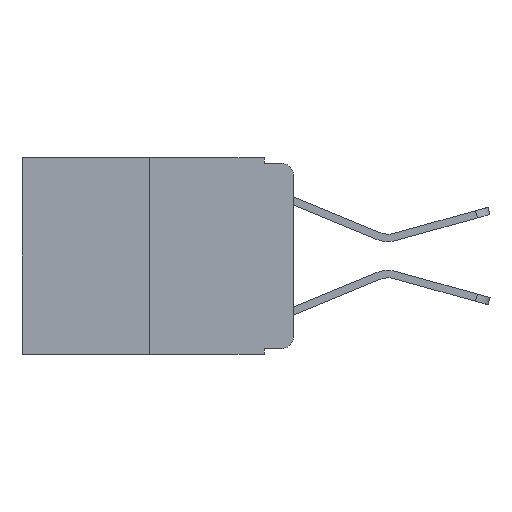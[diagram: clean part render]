
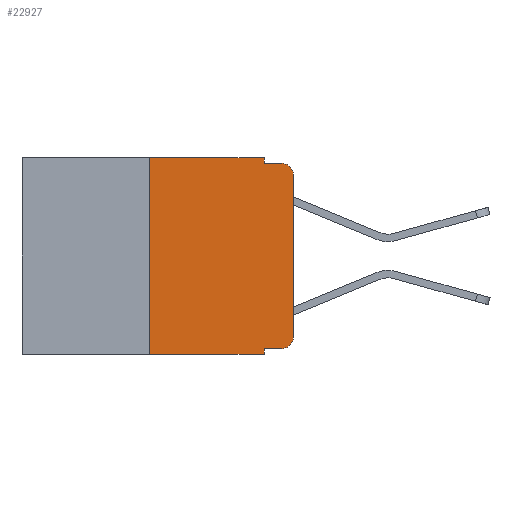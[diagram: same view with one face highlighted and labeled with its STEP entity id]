
A CAD part, left-side view. The second image highlights one B-rep face of the part: STEP entity #22927.
In plain terms, the highlighted planar face has unit normal (-1, 0, 0).
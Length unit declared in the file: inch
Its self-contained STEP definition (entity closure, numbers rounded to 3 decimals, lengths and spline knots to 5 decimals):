
#206 = EDGE_CURVE ( 'NONE', #16278, #2277, #17409, .T. ) ;
#449 = AXIS2_PLACEMENT_3D ( 'NONE', #2134, #2298, #22669 ) ;
#471 = ORIENTED_EDGE ( 'NONE', *, *, #9997, .T. ) ;
#782 = DIRECTION ( 'NONE',  ( 0., -1., 0. ) ) ;
#1039 = VERTEX_POINT ( 'NONE', #2807 ) ;
#1098 = DIRECTION ( 'NONE',  ( 1., 0., 0. ) ) ;
#1350 = CARTESIAN_POINT ( 'NONE',  ( 0., 0.051, 0. ) ) ;
#1511 = CIRCLE ( 'NONE', #449, 0.02 ) ;
#2094 = EDGE_CURVE ( 'NONE', #1039, #4390, #23998, .T. ) ;
#2134 = CARTESIAN_POINT ( 'NONE',  ( 0., 0.02, -0.313 ) ) ;
#2277 = VERTEX_POINT ( 'NONE', #12723 ) ;
#2298 = DIRECTION ( 'NONE',  ( -1., 0., 0. ) ) ;
#2807 = CARTESIAN_POINT ( 'NONE',  ( 0., 0.051, -0.333 ) ) ;
#3327 = VERTEX_POINT ( 'NONE', #22559 ) ;
#3357 = CARTESIAN_POINT ( 'NONE',  ( 0., 0.25, 0. ) ) ;
#3433 = VERTEX_POINT ( 'NONE', #19205 ) ;
#3616 = VECTOR ( 'NONE', #12734, 39.37008 ) ;
#4310 = EDGE_CURVE ( 'NONE', #16287, #16278, #10915, .T. ) ;
#4390 = VERTEX_POINT ( 'NONE', #21379 ) ;
#5100 = EDGE_CURVE ( 'NONE', #4390, #11190, #1511, .T. ) ;
#5334 = LINE ( 'NONE', #12309, #20200 ) ;
#5339 = VECTOR ( 'NONE', #16578, 39.37008 ) ;
#5647 = DIRECTION ( 'NONE',  ( 0., 0., -1. ) ) ;
#7017 = CARTESIAN_POINT ( 'NONE',  ( 0., 0.051, -0.333 ) ) ;
#7019 = VECTOR ( 'NONE', #22301, 39.37008 ) ;
#7652 = VECTOR ( 'NONE', #782, 39.37008 ) ;
#7689 = CARTESIAN_POINT ( 'NONE',  ( 0., 0.051, 0. ) ) ;
#8044 = ORIENTED_EDGE ( 'NONE', *, *, #22902, .F. ) ;
#8308 = VECTOR ( 'NONE', #10383, 39.37008 ) ;
#8868 = LINE ( 'NONE', #22062, #3616 ) ;
#9997 = EDGE_CURVE ( 'NONE', #11190, #17678, #17927, .T. ) ;
#9998 = VECTOR ( 'NONE', #16727, 39.37008 ) ;
#10328 = ORIENTED_EDGE ( 'NONE', *, *, #16482, .T. ) ;
#10383 = DIRECTION ( 'NONE',  ( 0., 0., 1. ) ) ;
#10706 = ORIENTED_EDGE ( 'NONE', *, *, #206, .F. ) ;
#10915 = LINE ( 'NONE', #15625, #7652 ) ;
#11114 = CARTESIAN_POINT ( 'NONE',  ( 0., 0., 0. ) ) ;
#11190 = VERTEX_POINT ( 'NONE', #12616 ) ;
#11338 = CARTESIAN_POINT ( 'NONE',  ( 0., 0.051, 0. ) ) ;
#11740 = LINE ( 'NONE', #11338, #7019 ) ;
#12203 = CARTESIAN_POINT ( 'NONE',  ( 0., 0.25, 0. ) ) ;
#12309 = CARTESIAN_POINT ( 'NONE',  ( 0., 0.473, -0.343 ) ) ;
#12383 = CIRCLE ( 'NONE', #13557, 0.02 ) ;
#12616 = CARTESIAN_POINT ( 'NONE',  ( 0., 0., -0.313 ) ) ;
#12723 = CARTESIAN_POINT ( 'NONE',  ( 0., 0.051, -0.01 ) ) ;
#12734 = DIRECTION ( 'NONE',  ( 0., -1., 0. ) ) ;
#13557 = AXIS2_PLACEMENT_3D ( 'NONE', #18805, #15183, #22638 ) ;
#15183 = DIRECTION ( 'NONE',  ( -1., 0., 0. ) ) ;
#15296 = ORIENTED_EDGE ( 'NONE', *, *, #16221, .T. ) ;
#15614 = CARTESIAN_POINT ( 'NONE',  ( 0., 0., -0.03 ) ) ;
#15625 = CARTESIAN_POINT ( 'NONE',  ( 0., 0.473, 0. ) ) ;
#15663 = EDGE_CURVE ( 'NONE', #2277, #3327, #8868, .T. ) ;
#15788 = CARTESIAN_POINT ( 'NONE',  ( 0., 0.473, 0. ) ) ;
#16036 = EDGE_LOOP ( 'NONE', ( #471, #10328, #18398, #10706, #16397, #8044, #15296, #20967, #22411, #17726 ) ) ;
#16221 = EDGE_CURVE ( 'NONE', #20838, #3433, #5334, .T. ) ;
#16278 = VERTEX_POINT ( 'NONE', #1350 ) ;
#16287 = VERTEX_POINT ( 'NONE', #3357 ) ;
#16397 = ORIENTED_EDGE ( 'NONE', *, *, #4310, .F. ) ;
#16482 = EDGE_CURVE ( 'NONE', #17678, #3327, #12383, .T. ) ;
#16578 = DIRECTION ( 'NONE',  ( 0., -1., 0. ) ) ;
#16727 = DIRECTION ( 'NONE',  ( 0., 0., 1. ) ) ;
#17409 = LINE ( 'NONE', #7689, #22945 ) ;
#17678 = VERTEX_POINT ( 'NONE', #15614 ) ;
#17726 = ORIENTED_EDGE ( 'NONE', *, *, #5100, .T. ) ;
#17884 = PLANE ( 'NONE',  #23952 ) ;
#17927 = LINE ( 'NONE', #11114, #9998 ) ;
#17963 = DIRECTION ( 'NONE',  ( 0., 0., -1. ) ) ;
#18252 = LINE ( 'NONE', #12203, #8308 ) ;
#18398 = ORIENTED_EDGE ( 'NONE', *, *, #15663, .F. ) ;
#18805 = CARTESIAN_POINT ( 'NONE',  ( 0., 0.02, -0.03 ) ) ;
#19198 = EDGE_CURVE ( 'NONE', #1039, #3433, #11740, .T. ) ;
#19205 = CARTESIAN_POINT ( 'NONE',  ( 0., 0.051, -0.343 ) ) ;
#20200 = VECTOR ( 'NONE', #23507, 39.37008 ) ;
#20838 = VERTEX_POINT ( 'NONE', #21889 ) ;
#20967 = ORIENTED_EDGE ( 'NONE', *, *, #19198, .F. ) ;
#21146 = FACE_OUTER_BOUND ( 'NONE', #16036, .T. ) ;
#21379 = CARTESIAN_POINT ( 'NONE',  ( 0., 0.02, -0.333 ) ) ;
#21889 = CARTESIAN_POINT ( 'NONE',  ( 0., 0.25, -0.343 ) ) ;
#22062 = CARTESIAN_POINT ( 'NONE',  ( 0., 0.051, -0.01 ) ) ;
#22301 = DIRECTION ( 'NONE',  ( 0., 0., -1. ) ) ;
#22411 = ORIENTED_EDGE ( 'NONE', *, *, #2094, .T. ) ;
#22559 = CARTESIAN_POINT ( 'NONE',  ( 0., 0.02, -0.01 ) ) ;
#22638 = DIRECTION ( 'NONE',  ( 0., 0., -1. ) ) ;
#22669 = DIRECTION ( 'NONE',  ( 0., 0., -1. ) ) ;
#22902 = EDGE_CURVE ( 'NONE', #20838, #16287, #18252, .T. ) ;
#22927 = ADVANCED_FACE ( 'NONE', ( #21146 ), #17884, .F. ) ;
#22945 = VECTOR ( 'NONE', #5647, 39.37008 ) ;
#23507 = DIRECTION ( 'NONE',  ( 0., -1., 0. ) ) ;
#23952 = AXIS2_PLACEMENT_3D ( 'NONE', #15788, #1098, #17963 ) ;
#23998 = LINE ( 'NONE', #7017, #5339 ) ;
